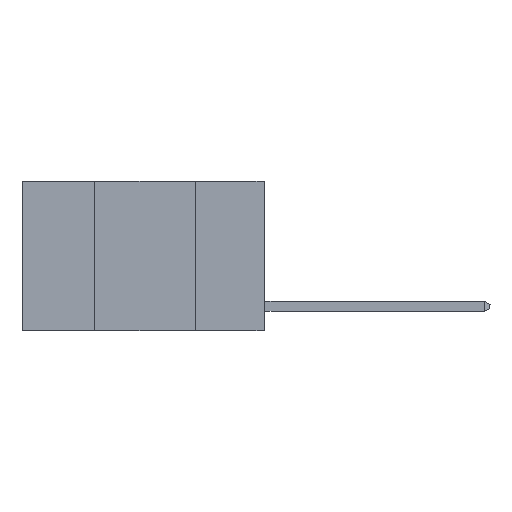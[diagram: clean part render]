
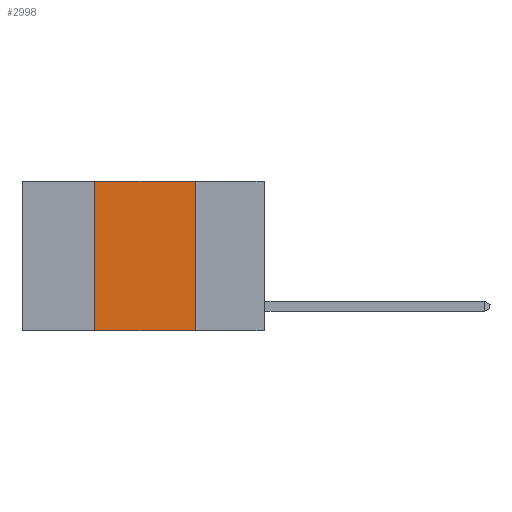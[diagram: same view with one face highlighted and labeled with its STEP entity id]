
A CAD part, left-side view. The second image highlights one B-rep face of the part: STEP entity #2998.
In plain terms, the highlighted planar face has unit normal (-1, 0, 0).
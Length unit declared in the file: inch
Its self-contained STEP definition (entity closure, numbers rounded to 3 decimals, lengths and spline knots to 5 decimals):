
#615 = CARTESIAN_POINT ( 'NONE',  ( 0., 0.17, -0.37 ) ) ;
#1621 = EDGE_LOOP ( 'NONE', ( #13296, #18485, #13903, #19145 ) ) ;
#1624 = AXIS2_PLACEMENT_3D ( 'NONE', #3271, #9487, #22457 ) ;
#2998 = ADVANCED_FACE ( 'NONE', ( #7111 ), #12740, .F. ) ;
#3091 = EDGE_CURVE ( 'NONE', #25284, #20683, #14516, .T. ) ;
#3271 = CARTESIAN_POINT ( 'NONE',  ( 0., 0.6, 0. ) ) ;
#3360 = CARTESIAN_POINT ( 'NONE',  ( 0., 0.6, -0.37 ) ) ;
#5288 = DIRECTION ( 'NONE',  ( 0., 0., 1. ) ) ;
#6866 = CARTESIAN_POINT ( 'NONE',  ( 0., 0.42, 0. ) ) ;
#7111 = FACE_OUTER_BOUND ( 'NONE', #1621, .T. ) ;
#7357 = DIRECTION ( 'NONE',  ( 0., -1., 0. ) ) ;
#9487 = DIRECTION ( 'NONE',  ( 1., 0., 0. ) ) ;
#12154 = EDGE_CURVE ( 'NONE', #22484, #20411, #24468, .T. ) ;
#12740 = PLANE ( 'NONE',  #1624 ) ;
#13150 = CARTESIAN_POINT ( 'NONE',  ( 0., 0.17, 0. ) ) ;
#13296 = ORIENTED_EDGE ( 'NONE', *, *, #15151, .F. ) ;
#13903 = ORIENTED_EDGE ( 'NONE', *, *, #24434, .F. ) ;
#14516 = LINE ( 'NONE', #3360, #25012 ) ;
#14824 = VECTOR ( 'NONE', #5288, 39.37008 ) ;
#15151 = EDGE_CURVE ( 'NONE', #20411, #20683, #16021, .T. ) ;
#16021 = LINE ( 'NONE', #13150, #20618 ) ;
#16112 = CARTESIAN_POINT ( 'NONE',  ( 0., 0.42, -0.37 ) ) ;
#17157 = CARTESIAN_POINT ( 'NONE',  ( 0., 0.42, 0. ) ) ;
#18485 = ORIENTED_EDGE ( 'NONE', *, *, #12154, .F. ) ;
#19145 = ORIENTED_EDGE ( 'NONE', *, *, #3091, .T. ) ;
#19457 = CARTESIAN_POINT ( 'NONE',  ( 0., 0.17, 0. ) ) ;
#20411 = VERTEX_POINT ( 'NONE', #19457 ) ;
#20606 = CARTESIAN_POINT ( 'NONE',  ( 0., 0.6, 0. ) ) ;
#20618 = VECTOR ( 'NONE', #24934, 39.37008 ) ;
#20670 = LINE ( 'NONE', #17157, #14824 ) ;
#20683 = VERTEX_POINT ( 'NONE', #615 ) ;
#22457 = DIRECTION ( 'NONE',  ( 0., 0., -1. ) ) ;
#22484 = VERTEX_POINT ( 'NONE', #6866 ) ;
#22615 = DIRECTION ( 'NONE',  ( 0., -1., 0. ) ) ;
#23858 = VECTOR ( 'NONE', #22615, 39.37008 ) ;
#24434 = EDGE_CURVE ( 'NONE', #25284, #22484, #20670, .T. ) ;
#24468 = LINE ( 'NONE', #20606, #23858 ) ;
#24934 = DIRECTION ( 'NONE',  ( 0., 0., -1. ) ) ;
#25012 = VECTOR ( 'NONE', #7357, 39.37008 ) ;
#25284 = VERTEX_POINT ( 'NONE', #16112 ) ;
